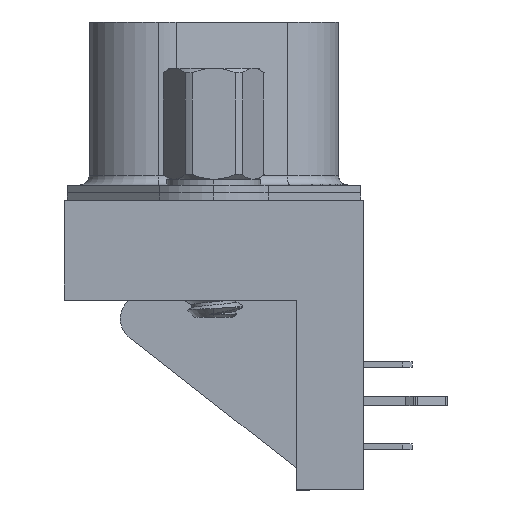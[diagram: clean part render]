
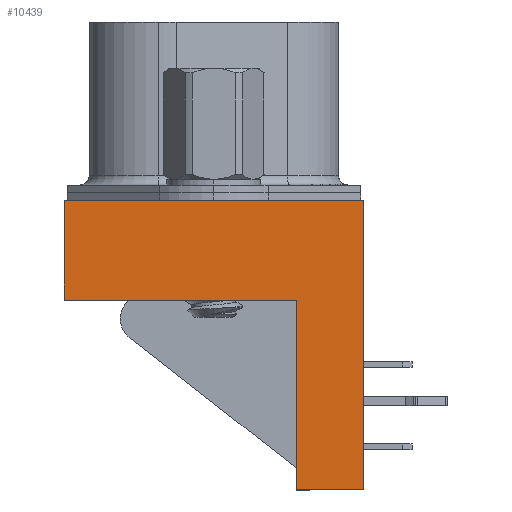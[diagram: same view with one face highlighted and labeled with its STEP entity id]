
A CAD part, left-side view. The second image highlights one B-rep face of the part: STEP entity #10439.
In plain terms, the highlighted planar face has unit normal (-1, 0, 0).
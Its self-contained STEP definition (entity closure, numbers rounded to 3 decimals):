
#1059 = LINE ( 'NONE', #87875, #59005 ) ;
#2028 = EDGE_CURVE ( 'NONE', #116724, #41519, #43486, .T. ) ;
#3259 = CARTESIAN_POINT ( 'NONE',  ( -4.125, -4.3, -15.1 ) ) ;
#4961 = FACE_OUTER_BOUND ( 'NONE', #89961, .T. ) ;
#5961 = LINE ( 'NONE', #119830, #93919 ) ;
#10439 = ADVANCED_FACE ( 'NONE', ( #4961 ), #47941, .T. ) ;
#15818 = CARTESIAN_POINT ( 'NONE',  ( -4.125, 7.8, 0. ) ) ;
#15950 = DIRECTION ( 'NONE',  ( 0., 0., 1. ) ) ;
#17428 = EDGE_CURVE ( 'NONE', #71865, #123740, #123322, .T. ) ;
#18091 = ORIENTED_EDGE ( 'NONE', *, *, #50436, .F. ) ;
#18643 = CARTESIAN_POINT ( 'NONE',  ( -4.125, -7.8, 0. ) ) ;
#22840 = EDGE_CURVE ( 'NONE', #41519, #43417, #5961, .T. ) ;
#24466 = VECTOR ( 'NONE', #117124, 1000. ) ;
#24824 = ORIENTED_EDGE ( 'NONE', *, *, #17428, .F. ) ;
#32060 = DIRECTION ( 'NONE',  ( 0., -1., 0. ) ) ;
#35692 = VERTEX_POINT ( 'NONE', #58348 ) ;
#35841 = DIRECTION ( 'NONE',  ( 0., 1., 0. ) ) ;
#41519 = VERTEX_POINT ( 'NONE', #126605 ) ;
#42124 = ORIENTED_EDGE ( 'NONE', *, *, #78206, .T. ) ;
#43417 = VERTEX_POINT ( 'NONE', #161702 ) ;
#43486 = LINE ( 'NONE', #3259, #24466 ) ;
#43915 = LINE ( 'NONE', #182920, #113110 ) ;
#47941 = PLANE ( 'NONE',  #90512 ) ;
#50436 = EDGE_CURVE ( 'NONE', #43417, #71865, #43915, .T. ) ;
#56645 = LINE ( 'NONE', #127530, #144024 ) ;
#58348 = CARTESIAN_POINT ( 'NONE',  ( -4.125, -7.8, -15.1 ) ) ;
#59005 = VECTOR ( 'NONE', #15950, 1000. ) ;
#67117 = ORIENTED_EDGE ( 'NONE', *, *, #2028, .F. ) ;
#71865 = VERTEX_POINT ( 'NONE', #15818 ) ;
#78206 = EDGE_CURVE ( 'NONE', #35692, #123740, #1059, .T. ) ;
#87875 = CARTESIAN_POINT ( 'NONE',  ( -4.125, -7.8, -15.1 ) ) ;
#89954 = CARTESIAN_POINT ( 'NONE',  ( -4.125, 7.8, -15.1 ) ) ;
#89961 = EDGE_LOOP ( 'NONE', ( #119253, #67117, #138636, #42124, #24824, #18091 ) ) ;
#90512 = AXIS2_PLACEMENT_3D ( 'NONE', #89954, #146806, #32060 ) ;
#93919 = VECTOR ( 'NONE', #35841, 1000. ) ;
#96248 = DIRECTION ( 'NONE',  ( 0., -1., 0. ) ) ;
#98079 = DIRECTION ( 'NONE',  ( 0., 0., 1. ) ) ;
#113110 = VECTOR ( 'NONE', #98079, 1000. ) ;
#113768 = EDGE_CURVE ( 'NONE', #116724, #35692, #56645, .T. ) ;
#116724 = VERTEX_POINT ( 'NONE', #175981 ) ;
#117124 = DIRECTION ( 'NONE',  ( 0., 0., 1. ) ) ;
#119253 = ORIENTED_EDGE ( 'NONE', *, *, #22840, .F. ) ;
#119830 = CARTESIAN_POINT ( 'NONE',  ( -4.125, 7.8, -5.2 ) ) ;
#123322 = LINE ( 'NONE', #153097, #154386 ) ;
#123740 = VERTEX_POINT ( 'NONE', #18643 ) ;
#125661 = DIRECTION ( 'NONE',  ( 0., -1., 0. ) ) ;
#126605 = CARTESIAN_POINT ( 'NONE',  ( -4.125, -4.3, -5.2 ) ) ;
#127530 = CARTESIAN_POINT ( 'NONE',  ( -4.125, 7.8, -15.1 ) ) ;
#138636 = ORIENTED_EDGE ( 'NONE', *, *, #113768, .T. ) ;
#144024 = VECTOR ( 'NONE', #125661, 1000. ) ;
#146806 = DIRECTION ( 'NONE',  ( -1., 0., 0. ) ) ;
#153097 = CARTESIAN_POINT ( 'NONE',  ( -4.125, 7.8, 0. ) ) ;
#154386 = VECTOR ( 'NONE', #96248, 1000. ) ;
#161702 = CARTESIAN_POINT ( 'NONE',  ( -4.125, 7.8, -5.2 ) ) ;
#175981 = CARTESIAN_POINT ( 'NONE',  ( -4.125, -4.3, -15.1 ) ) ;
#182920 = CARTESIAN_POINT ( 'NONE',  ( -4.125, 7.8, -15.1 ) ) ;
